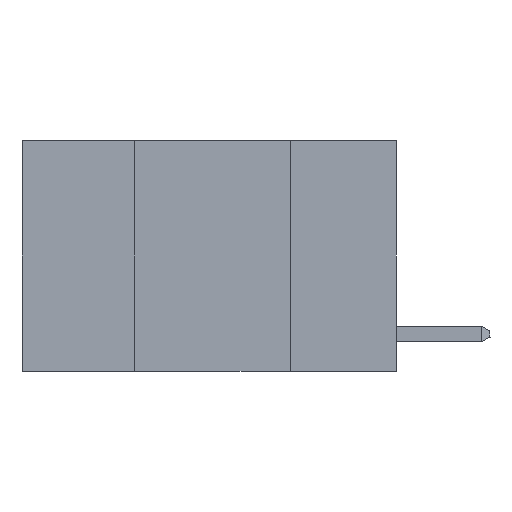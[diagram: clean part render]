
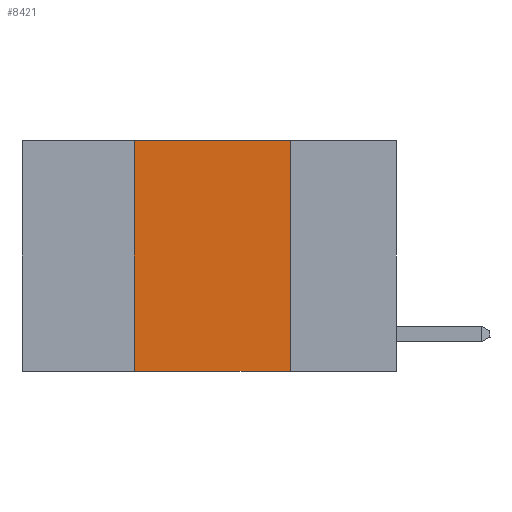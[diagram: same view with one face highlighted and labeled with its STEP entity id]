
A CAD part, left-side view. The second image highlights one B-rep face of the part: STEP entity #8421.
In plain terms, the highlighted planar face has unit normal (-1, 0, 0).
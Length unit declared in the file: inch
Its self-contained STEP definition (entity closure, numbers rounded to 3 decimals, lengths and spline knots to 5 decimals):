
#1084 = CARTESIAN_POINT ( 'NONE',  ( 0., 0.42, 0. ) ) ;
#1507 = VERTEX_POINT ( 'NONE', #13541 ) ;
#1610 = EDGE_CURVE ( 'NONE', #1507, #15205, #5782, .T. ) ;
#1616 = EDGE_CURVE ( 'NONE', #1507, #1955, #8891, .T. ) ;
#1645 = EDGE_CURVE ( 'NONE', #7083, #15205, #7934, .T. ) ;
#1792 = FACE_OUTER_BOUND ( 'NONE', #2333, .T. ) ;
#1955 = VERTEX_POINT ( 'NONE', #1084 ) ;
#2326 = EDGE_CURVE ( 'NONE', #1955, #7083, #15344, .T. ) ;
#2333 = EDGE_LOOP ( 'NONE', ( #8034, #13403, #6393, #10967 ) ) ;
#2737 = AXIS2_PLACEMENT_3D ( 'NONE', #8985, #19660, #10538 ) ;
#4694 = CARTESIAN_POINT ( 'NONE',  ( 0., 0.42, 0. ) ) ;
#4845 = VECTOR ( 'NONE', #7677, 39.37008 ) ;
#5782 = LINE ( 'NONE', #18390, #4845 ) ;
#6393 = ORIENTED_EDGE ( 'NONE', *, *, #1616, .F. ) ;
#7083 = VERTEX_POINT ( 'NONE', #7881 ) ;
#7298 = CARTESIAN_POINT ( 'NONE',  ( 0., 0.6, 0. ) ) ;
#7677 = DIRECTION ( 'NONE',  ( 0., -1., 0. ) ) ;
#7881 = CARTESIAN_POINT ( 'NONE',  ( 0., 0.17, 0. ) ) ;
#7934 = LINE ( 'NONE', #9347, #12029 ) ;
#8034 = ORIENTED_EDGE ( 'NONE', *, *, #1645, .F. ) ;
#8421 = ADVANCED_FACE ( 'NONE', ( #1792 ), #16625, .F. ) ;
#8891 = LINE ( 'NONE', #4694, #16570 ) ;
#8985 = CARTESIAN_POINT ( 'NONE',  ( 0., 0.6, 0. ) ) ;
#9347 = CARTESIAN_POINT ( 'NONE',  ( 0., 0.17, 0. ) ) ;
#10491 = CARTESIAN_POINT ( 'NONE',  ( 0., 0.17, -0.37 ) ) ;
#10538 = DIRECTION ( 'NONE',  ( 0., 0., -1. ) ) ;
#10967 = ORIENTED_EDGE ( 'NONE', *, *, #1610, .T. ) ;
#12029 = VECTOR ( 'NONE', #20032, 39.37008 ) ;
#12320 = DIRECTION ( 'NONE',  ( 0., 0., 1. ) ) ;
#13403 = ORIENTED_EDGE ( 'NONE', *, *, #2326, .F. ) ;
#13541 = CARTESIAN_POINT ( 'NONE',  ( 0., 0.42, -0.37 ) ) ;
#14893 = DIRECTION ( 'NONE',  ( 0., -1., 0. ) ) ;
#15205 = VERTEX_POINT ( 'NONE', #10491 ) ;
#15344 = LINE ( 'NONE', #7298, #18877 ) ;
#16570 = VECTOR ( 'NONE', #12320, 39.37008 ) ;
#16625 = PLANE ( 'NONE',  #2737 ) ;
#18390 = CARTESIAN_POINT ( 'NONE',  ( 0., 0.6, -0.37 ) ) ;
#18877 = VECTOR ( 'NONE', #14893, 39.37008 ) ;
#19660 = DIRECTION ( 'NONE',  ( 1., 0., 0. ) ) ;
#20032 = DIRECTION ( 'NONE',  ( 0., 0., -1. ) ) ;
